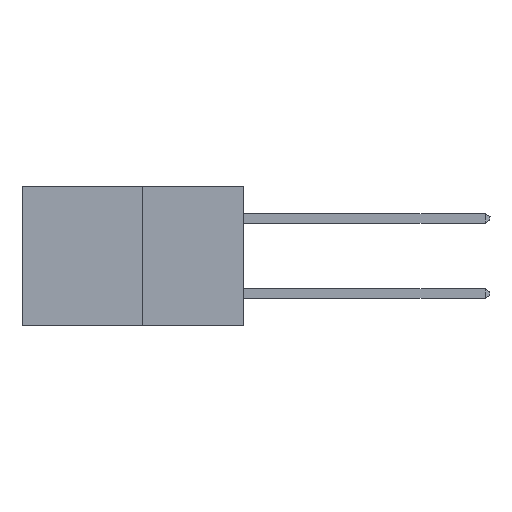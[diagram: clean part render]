
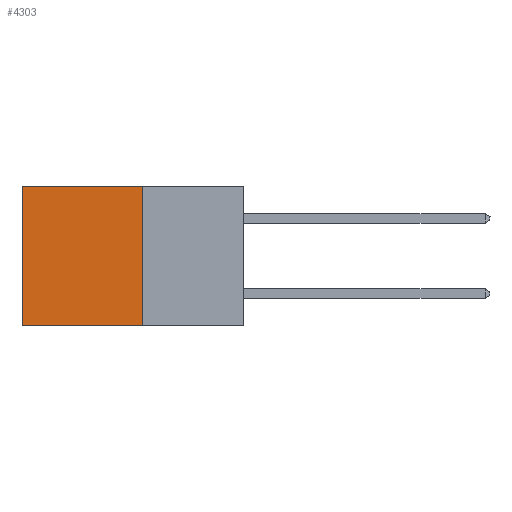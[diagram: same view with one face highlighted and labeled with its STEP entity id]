
A CAD part, left-side view. The second image highlights one B-rep face of the part: STEP entity #4303.
In plain terms, the highlighted planar face has unit normal (-1, 0, 0).
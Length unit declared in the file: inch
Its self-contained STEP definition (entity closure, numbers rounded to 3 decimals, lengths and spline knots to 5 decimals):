
#381 = ORIENTED_EDGE ( 'NONE', *, *, #1018, .F. ) ;
#587 = CARTESIAN_POINT ( 'NONE',  ( 0.277, 0.59, 0. ) ) ;
#798 = DIRECTION ( 'NONE',  ( 0., 0., -1. ) ) ;
#808 = CARTESIAN_POINT ( 'NONE',  ( 0.277, 0.59, -0.37 ) ) ;
#1018 = EDGE_CURVE ( 'NONE', #6374, #5309, #2849, .T. ) ;
#1240 = VECTOR ( 'NONE', #1997, 39.37008 ) ;
#1864 = CARTESIAN_POINT ( 'NONE',  ( 0.277, 0.27, -0.37 ) ) ;
#1997 = DIRECTION ( 'NONE',  ( 0., 1., 0. ) ) ;
#2550 = VERTEX_POINT ( 'NONE', #587 ) ;
#2849 = LINE ( 'NONE', #7272, #5252 ) ;
#2983 = VECTOR ( 'NONE', #3682, 39.37008 ) ;
#3218 = ORIENTED_EDGE ( 'NONE', *, *, #11945, .F. ) ;
#3682 = DIRECTION ( 'NONE',  ( 0., 1., 0. ) ) ;
#3982 = CARTESIAN_POINT ( 'NONE',  ( 0.277, 0.27, 0. ) ) ;
#4303 = ADVANCED_FACE ( 'NONE', ( #9650 ), #8082, .F. ) ;
#5043 = CARTESIAN_POINT ( 'NONE',  ( 0.277, 0.27, 0. ) ) ;
#5182 = CARTESIAN_POINT ( 'NONE',  ( 0.277, 0.59, -0.37 ) ) ;
#5252 = VECTOR ( 'NONE', #8239, 39.37008 ) ;
#5309 = VERTEX_POINT ( 'NONE', #1864 ) ;
#5473 = EDGE_CURVE ( 'NONE', #2550, #7873, #7035, .T. ) ;
#6374 = VERTEX_POINT ( 'NONE', #3982 ) ;
#6423 = EDGE_CURVE ( 'NONE', #6374, #2550, #9402, .T. ) ;
#7035 = LINE ( 'NONE', #808, #9762 ) ;
#7272 = CARTESIAN_POINT ( 'NONE',  ( 0.277, 0.27, -0.37 ) ) ;
#7638 = AXIS2_PLACEMENT_3D ( 'NONE', #8072, #8031, #8016 ) ;
#7873 = VERTEX_POINT ( 'NONE', #5182 ) ;
#8016 = DIRECTION ( 'NONE',  ( 0., 0., -1. ) ) ;
#8031 = DIRECTION ( 'NONE',  ( 1., 0., 0. ) ) ;
#8072 = CARTESIAN_POINT ( 'NONE',  ( 0.277, 0.27, -0.37 ) ) ;
#8082 = PLANE ( 'NONE',  #7638 ) ;
#8239 = DIRECTION ( 'NONE',  ( 0., 0., -1. ) ) ;
#8774 = CARTESIAN_POINT ( 'NONE',  ( 0.277, 0.27, -0.37 ) ) ;
#9402 = LINE ( 'NONE', #5043, #1240 ) ;
#9650 = FACE_OUTER_BOUND ( 'NONE', #12358, .T. ) ;
#9762 = VECTOR ( 'NONE', #798, 39.37008 ) ;
#11123 = LINE ( 'NONE', #8774, #2983 ) ;
#11534 = ORIENTED_EDGE ( 'NONE', *, *, #5473, .T. ) ;
#11869 = ORIENTED_EDGE ( 'NONE', *, *, #6423, .T. ) ;
#11945 = EDGE_CURVE ( 'NONE', #5309, #7873, #11123, .T. ) ;
#12358 = EDGE_LOOP ( 'NONE', ( #11534, #3218, #381, #11869 ) ) ;
